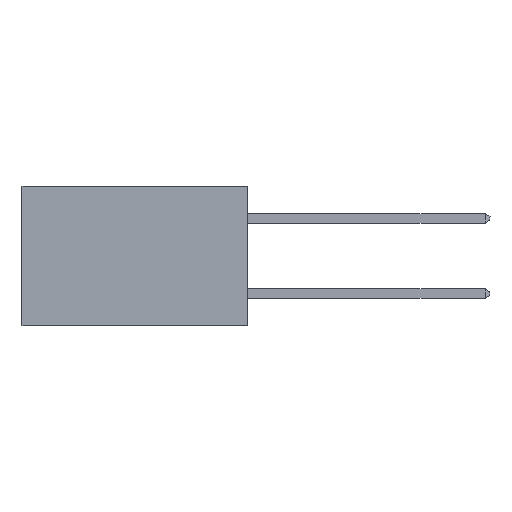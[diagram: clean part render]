
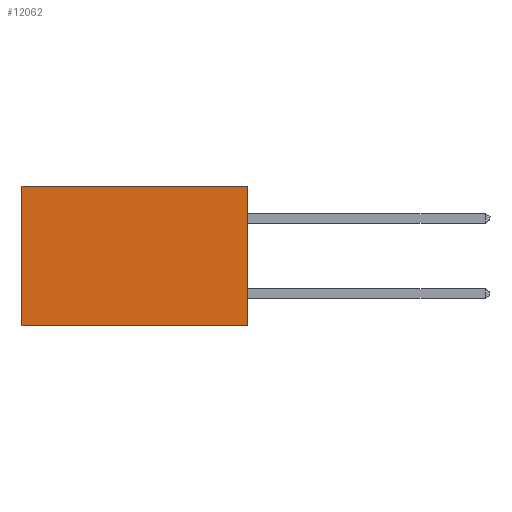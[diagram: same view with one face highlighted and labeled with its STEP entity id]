
A CAD part, left-side view. The second image highlights one B-rep face of the part: STEP entity #12062.
In plain terms, the highlighted planar face has unit normal (-1, 0, 0).
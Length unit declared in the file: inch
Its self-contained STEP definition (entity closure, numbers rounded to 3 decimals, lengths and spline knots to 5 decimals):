
#344 = VECTOR ( 'NONE', #8358, 39.37008 ) ;
#633 = CARTESIAN_POINT ( 'NONE',  ( 0.2615, 0., -0.37 ) ) ;
#2005 = CARTESIAN_POINT ( 'NONE',  ( 0.2615, 0.6, -0.37 ) ) ;
#2314 = ORIENTED_EDGE ( 'NONE', *, *, #5829, .F. ) ;
#2598 = LINE ( 'NONE', #5906, #11378 ) ;
#2615 = CARTESIAN_POINT ( 'NONE',  ( 0.2615, 0.6, 0. ) ) ;
#2904 = CARTESIAN_POINT ( 'NONE',  ( 0.2615, 0., 0. ) ) ;
#3064 = ORIENTED_EDGE ( 'NONE', *, *, #12013, .T. ) ;
#3346 = DIRECTION ( 'NONE',  ( 1., 0., 0. ) ) ;
#3712 = ORIENTED_EDGE ( 'NONE', *, *, #7603, .F. ) ;
#4417 = VECTOR ( 'NONE', #5211, 39.37008 ) ;
#4797 = VECTOR ( 'NONE', #8247, 39.37008 ) ;
#5064 = CARTESIAN_POINT ( 'NONE',  ( 0.2615, 0., 0. ) ) ;
#5074 = LINE ( 'NONE', #2904, #4417 ) ;
#5211 = DIRECTION ( 'NONE',  ( 0., 1., 0. ) ) ;
#5366 = VERTEX_POINT ( 'NONE', #2615 ) ;
#5829 = EDGE_CURVE ( 'NONE', #6350, #13044, #2598, .T. ) ;
#5906 = CARTESIAN_POINT ( 'NONE',  ( 0.2615, 0., -0.37 ) ) ;
#6350 = VERTEX_POINT ( 'NONE', #5064 ) ;
#6523 = FACE_OUTER_BOUND ( 'NONE', #13560, .T. ) ;
#7374 = LINE ( 'NONE', #2005, #344 ) ;
#7603 = EDGE_CURVE ( 'NONE', #13044, #9941, #10300, .T. ) ;
#7792 = DIRECTION ( 'NONE',  ( 0., 0., -1. ) ) ;
#8056 = CARTESIAN_POINT ( 'NONE',  ( 0.2615, 0.6, -0.37 ) ) ;
#8247 = DIRECTION ( 'NONE',  ( 0., 1., 0. ) ) ;
#8358 = DIRECTION ( 'NONE',  ( 0., 0., -1. ) ) ;
#8599 = ORIENTED_EDGE ( 'NONE', *, *, #12912, .T. ) ;
#8763 = CARTESIAN_POINT ( 'NONE',  ( 0.2615, 0., -0.37 ) ) ;
#9941 = VERTEX_POINT ( 'NONE', #8056 ) ;
#10300 = LINE ( 'NONE', #633, #4797 ) ;
#10778 = CARTESIAN_POINT ( 'NONE',  ( 0.2615, 0., -0.37 ) ) ;
#11378 = VECTOR ( 'NONE', #7792, 39.37008 ) ;
#11869 = AXIS2_PLACEMENT_3D ( 'NONE', #8763, #3346, #12112 ) ;
#12013 = EDGE_CURVE ( 'NONE', #5366, #9941, #7374, .T. ) ;
#12041 = PLANE ( 'NONE',  #11869 ) ;
#12062 = ADVANCED_FACE ( 'NONE', ( #6523 ), #12041, .F. ) ;
#12112 = DIRECTION ( 'NONE',  ( 0., 0., -1. ) ) ;
#12912 = EDGE_CURVE ( 'NONE', #6350, #5366, #5074, .T. ) ;
#13044 = VERTEX_POINT ( 'NONE', #10778 ) ;
#13560 = EDGE_LOOP ( 'NONE', ( #3064, #3712, #2314, #8599 ) ) ;
